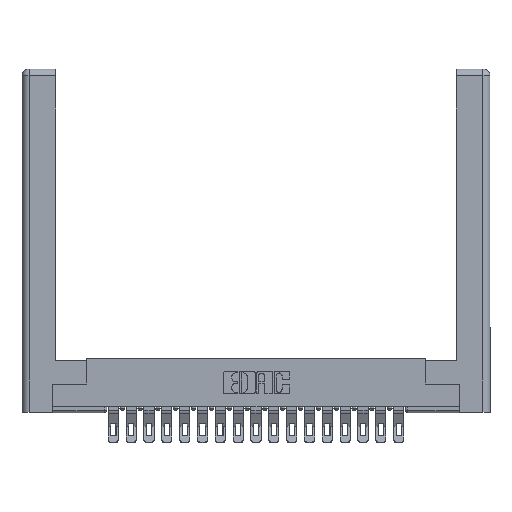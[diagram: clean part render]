
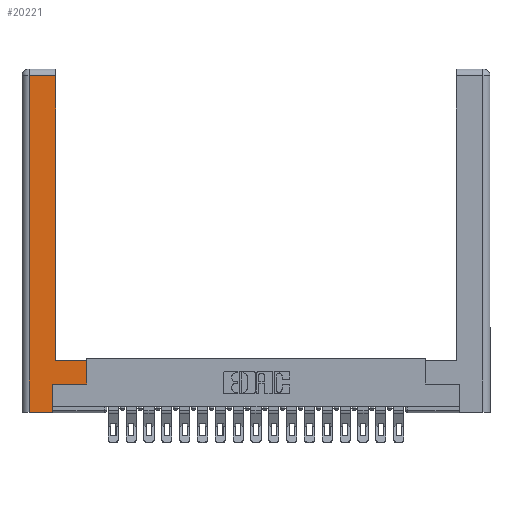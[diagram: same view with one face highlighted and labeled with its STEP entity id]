
A CAD part, top view. The second image highlights one B-rep face of the part: STEP entity #20221.
In plain terms, the highlighted planar face has unit normal (0, 0, 1).
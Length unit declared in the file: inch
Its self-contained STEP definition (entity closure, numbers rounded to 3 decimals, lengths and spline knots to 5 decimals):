
#768 = VECTOR ( 'NONE', #15210, 39.37008 ) ;
#839 = CARTESIAN_POINT ( 'NONE',  ( 0.295, 2.94, 0. ) ) ;
#1200 = EDGE_CURVE ( 'NONE', #19103, #3805, #19515, .T. ) ;
#1297 = CARTESIAN_POINT ( 'NONE',  ( 0.265, 0., 0. ) ) ;
#1776 = DIRECTION ( 'NONE',  ( 0., 1., 0. ) ) ;
#1829 = DIRECTION ( 'NONE',  ( -1., 0., 0. ) ) ;
#1953 = ORIENTED_EDGE ( 'NONE', *, *, #12906, .T. ) ;
#1990 = ORIENTED_EDGE ( 'NONE', *, *, #11901, .T. ) ;
#2523 = DIRECTION ( 'NONE',  ( 0., -1., 0. ) ) ;
#2726 = CARTESIAN_POINT ( 'NONE',  ( 0.0615, 2.94, 0. ) ) ;
#2972 = EDGE_CURVE ( 'NONE', #3805, #4291, #3683, .T. ) ;
#3269 = DIRECTION ( 'NONE',  ( -1., 0., 0. ) ) ;
#3683 = LINE ( 'NONE', #20021, #18110 ) ;
#3792 = CARTESIAN_POINT ( 'NONE',  ( 0.265, 0.245, 0. ) ) ;
#3805 = VERTEX_POINT ( 'NONE', #17342 ) ;
#4291 = VERTEX_POINT ( 'NONE', #1297 ) ;
#4520 = DIRECTION ( 'NONE',  ( 0., 1., 0. ) ) ;
#4871 = ORIENTED_EDGE ( 'NONE', *, *, #12141, .T. ) ;
#5198 = DIRECTION ( 'NONE',  ( 1., 0., 0. ) ) ;
#6422 = CARTESIAN_POINT ( 'NONE',  ( 0.565, 0.245, 0. ) ) ;
#6654 = DIRECTION ( 'NONE',  ( -1., 0., 0. ) ) ;
#7046 = DIRECTION ( 'NONE',  ( 0., 0., -1. ) ) ;
#7162 = PLANE ( 'NONE',  #10955 ) ;
#7809 = CARTESIAN_POINT ( 'NONE',  ( 0.295, 0.45, 0. ) ) ;
#7900 = ORIENTED_EDGE ( 'NONE', *, *, #11843, .T. ) ;
#8294 = VERTEX_POINT ( 'NONE', #6422 ) ;
#9830 = CARTESIAN_POINT ( 'NONE',  ( 0.0615, 2.94, 0. ) ) ;
#9873 = CARTESIAN_POINT ( 'NONE',  ( 0.565, 0.45, 0. ) ) ;
#9994 = LINE ( 'NONE', #14760, #19132 ) ;
#10141 = VERTEX_POINT ( 'NONE', #3792 ) ;
#10770 = DIRECTION ( 'NONE',  ( 1., 0., 0. ) ) ;
#10804 = VERTEX_POINT ( 'NONE', #9873 ) ;
#10836 = ORIENTED_EDGE ( 'NONE', *, *, #17631, .T. ) ;
#10955 = AXIS2_PLACEMENT_3D ( 'NONE', #13132, #7046, #6654 ) ;
#11098 = LINE ( 'NONE', #15977, #17675 ) ;
#11842 = VECTOR ( 'NONE', #1829, 39.37008 ) ;
#11843 = EDGE_CURVE ( 'NONE', #8294, #10804, #11098, .T. ) ;
#11901 = EDGE_CURVE ( 'NONE', #10141, #8294, #12426, .T. ) ;
#11911 = VERTEX_POINT ( 'NONE', #839 ) ;
#12141 = EDGE_CURVE ( 'NONE', #13612, #11911, #14206, .T. ) ;
#12426 = LINE ( 'NONE', #19117, #12841 ) ;
#12702 = CARTESIAN_POINT ( 'NONE',  ( 0.0615, 0., 0. ) ) ;
#12841 = VECTOR ( 'NONE', #10770, 39.37008 ) ;
#12906 = EDGE_CURVE ( 'NONE', #11911, #19103, #13285, .T. ) ;
#13132 = CARTESIAN_POINT ( 'NONE',  ( 0., 0., 0. ) ) ;
#13285 = LINE ( 'NONE', #9830, #11842 ) ;
#13517 = EDGE_LOOP ( 'NONE', ( #4871, #1953, #19429, #15472, #14705, #1990, #7900, #10836 ) ) ;
#13612 = VERTEX_POINT ( 'NONE', #14235 ) ;
#13750 = EDGE_CURVE ( 'NONE', #4291, #10141, #9994, .T. ) ;
#14206 = LINE ( 'NONE', #15830, #768 ) ;
#14235 = CARTESIAN_POINT ( 'NONE',  ( 0.295, 0.45, 0. ) ) ;
#14705 = ORIENTED_EDGE ( 'NONE', *, *, #13750, .T. ) ;
#14760 = CARTESIAN_POINT ( 'NONE',  ( 0.265, 0.245, 0. ) ) ;
#15210 = DIRECTION ( 'NONE',  ( 0., 1., 0. ) ) ;
#15472 = ORIENTED_EDGE ( 'NONE', *, *, #2972, .T. ) ;
#15830 = CARTESIAN_POINT ( 'NONE',  ( 0.295, 3., 0. ) ) ;
#15977 = CARTESIAN_POINT ( 'NONE',  ( 0.565, 0.45, 0. ) ) ;
#16507 = FACE_OUTER_BOUND ( 'NONE', #13517, .T. ) ;
#16611 = VECTOR ( 'NONE', #2523, 39.37008 ) ;
#17342 = CARTESIAN_POINT ( 'NONE',  ( 0.0615, 0., 0. ) ) ;
#17631 = EDGE_CURVE ( 'NONE', #10804, #13612, #21129, .T. ) ;
#17675 = VECTOR ( 'NONE', #4520, 39.37008 ) ;
#18110 = VECTOR ( 'NONE', #5198, 39.37008 ) ;
#19103 = VERTEX_POINT ( 'NONE', #2726 ) ;
#19117 = CARTESIAN_POINT ( 'NONE',  ( 0.565, 0.245, 0. ) ) ;
#19132 = VECTOR ( 'NONE', #1776, 39.37008 ) ;
#19429 = ORIENTED_EDGE ( 'NONE', *, *, #1200, .T. ) ;
#19515 = LINE ( 'NONE', #12702, #16611 ) ;
#20021 = CARTESIAN_POINT ( 'NONE',  ( 0.265, 0., 0. ) ) ;
#20221 = ADVANCED_FACE ( 'NONE', ( #16507 ), #7162, .F. ) ;
#20946 = VECTOR ( 'NONE', #3269, 39.37008 ) ;
#21129 = LINE ( 'NONE', #7809, #20946 ) ;
